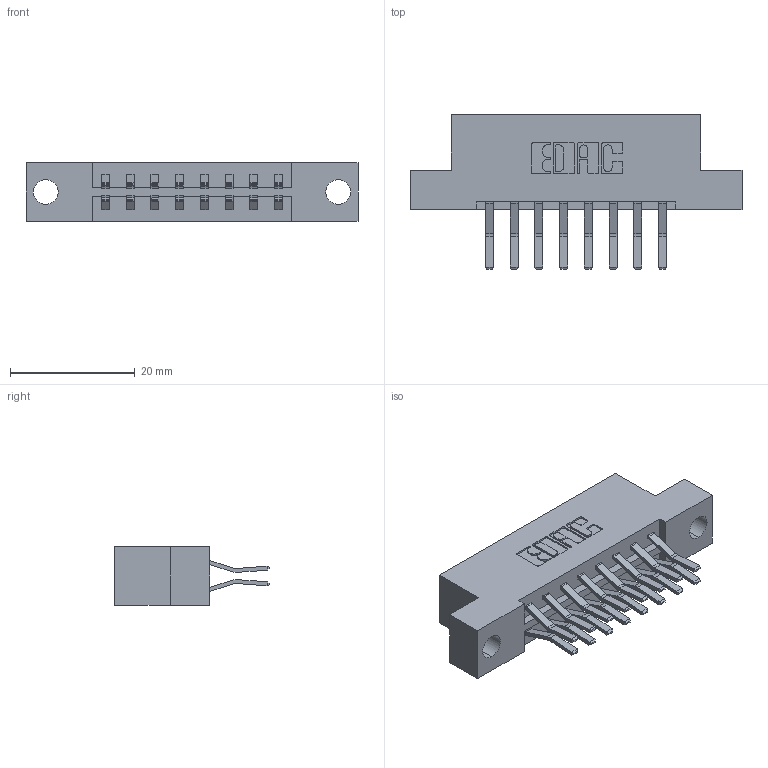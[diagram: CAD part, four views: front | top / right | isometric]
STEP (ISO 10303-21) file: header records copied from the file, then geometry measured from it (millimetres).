
FILE_DESCRIPTION (( 'STEP AP203' ), '1' );
FILE_NAME ('833-016-560-204.STEP', '2020-05-31T19:19:32', ( '' ), ( '' ), 'SwSTEP 2.0', 'SolidWorks 2020', '' );
FILE_SCHEMA (( 'CONFIG_CONTROL_DESIGN' ));
Length unit declared in the file: inch
Products named in the file (3): 345-292-001_560 Tail; 833-016-560-204; 833 Part_Flush - .156 Dia - TH
Assembly tree (17 placements, depth 2):
  833-016-560-204
    833 Part_Flush - .156 Dia - TH
    345-292-001_560 Tail  x16
Bounding box: 53.24 x 24.78 x 9.4 mm (x, y, z)
Volume: 5134.4 mm3; surface area: 5803.4 mm2
Topology: 17 solids, 17 shells, 978 faces, 2887 edges, 1902 vertices
Faces by surface type: plane 646, cylinder 332
Entity records: 9635 total; most frequent: CARTESIAN_POINT 1638, ORIENTED_EDGE 1574, DIRECTION 1463, EDGE_CURVE 787, LINE 655, VECTOR 655, VERTEX_POINT 522, AXIS2_PLACEMENT_3D 404
